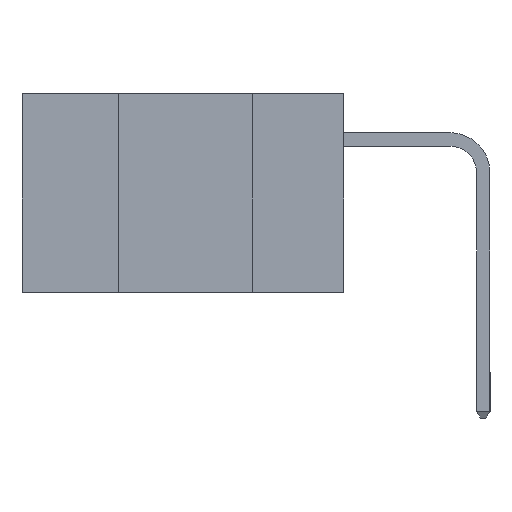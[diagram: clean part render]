
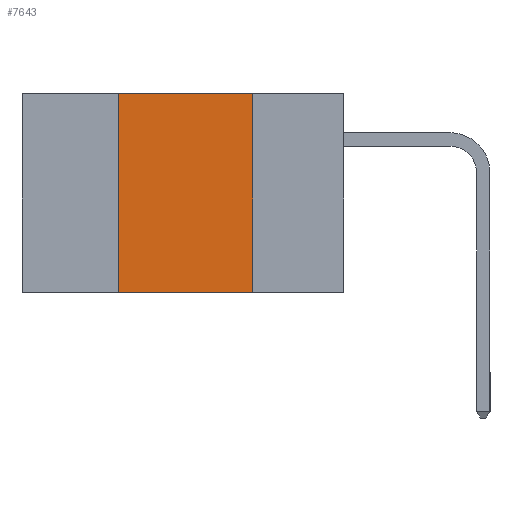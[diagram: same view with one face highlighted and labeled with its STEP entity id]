
A CAD part, left-side view. The second image highlights one B-rep face of the part: STEP entity #7643.
In plain terms, the highlighted planar face has unit normal (-1, 0, 0).
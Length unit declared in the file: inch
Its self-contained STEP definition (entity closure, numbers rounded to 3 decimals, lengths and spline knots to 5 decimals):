
#184 = DIRECTION ( 'NONE',  ( 0., 0., -1. ) ) ;
#296 = DIRECTION ( 'NONE',  ( 0., 0., 1. ) ) ;
#327 = EDGE_CURVE ( 'NONE', #404, #3056, #442, .T. ) ;
#369 = VECTOR ( 'NONE', #184, 39.37008 ) ;
#404 = VERTEX_POINT ( 'NONE', #1425 ) ;
#442 = LINE ( 'NONE', #5230, #5827 ) ;
#724 = DIRECTION ( 'NONE',  ( 1., 0., 0. ) ) ;
#974 = ORIENTED_EDGE ( 'NONE', *, *, #4785, .F. ) ;
#1425 = CARTESIAN_POINT ( 'NONE',  ( 0., 0.42, -0.37 ) ) ;
#1673 = LINE ( 'NONE', #6516, #4707 ) ;
#1913 = ORIENTED_EDGE ( 'NONE', *, *, #327, .T. ) ;
#2406 = LINE ( 'NONE', #7204, #369 ) ;
#2574 = ORIENTED_EDGE ( 'NONE', *, *, #10023, .F. ) ;
#2920 = DIRECTION ( 'NONE',  ( 0., -1., 0. ) ) ;
#2927 = CARTESIAN_POINT ( 'NONE',  ( 0., 0.17, -0.37 ) ) ;
#2945 = PLANE ( 'NONE',  #4422 ) ;
#3056 = VERTEX_POINT ( 'NONE', #2927 ) ;
#3725 = CARTESIAN_POINT ( 'NONE',  ( 0., 0.6, 0. ) ) ;
#3873 = EDGE_CURVE ( 'NONE', #8000, #7062, #1673, .T. ) ;
#4307 = LINE ( 'NONE', #8079, #5428 ) ;
#4375 = CARTESIAN_POINT ( 'NONE',  ( 0., 0.17, 0. ) ) ;
#4422 = AXIS2_PLACEMENT_3D ( 'NONE', #3725, #724, #8637 ) ;
#4568 = FACE_OUTER_BOUND ( 'NONE', #7831, .T. ) ;
#4707 = VECTOR ( 'NONE', #7996, 39.37008 ) ;
#4785 = EDGE_CURVE ( 'NONE', #7062, #3056, #2406, .T. ) ;
#5230 = CARTESIAN_POINT ( 'NONE',  ( 0., 0.6, -0.37 ) ) ;
#5428 = VECTOR ( 'NONE', #296, 39.37008 ) ;
#5827 = VECTOR ( 'NONE', #2920, 39.37008 ) ;
#5974 = CARTESIAN_POINT ( 'NONE',  ( 0., 0.42, 0. ) ) ;
#6516 = CARTESIAN_POINT ( 'NONE',  ( 0., 0.6, 0. ) ) ;
#7062 = VERTEX_POINT ( 'NONE', #4375 ) ;
#7204 = CARTESIAN_POINT ( 'NONE',  ( 0., 0.17, -0.37 ) ) ;
#7643 = ADVANCED_FACE ( 'NONE', ( #4568 ), #2945, .F. ) ;
#7831 = EDGE_LOOP ( 'NONE', ( #974, #9845, #2574, #1913 ) ) ;
#7996 = DIRECTION ( 'NONE',  ( 0., -1., 0. ) ) ;
#8000 = VERTEX_POINT ( 'NONE', #5974 ) ;
#8079 = CARTESIAN_POINT ( 'NONE',  ( 0., 0.42, -0.37 ) ) ;
#8637 = DIRECTION ( 'NONE',  ( 0., 0., -1. ) ) ;
#9845 = ORIENTED_EDGE ( 'NONE', *, *, #3873, .F. ) ;
#10023 = EDGE_CURVE ( 'NONE', #404, #8000, #4307, .T. ) ;
